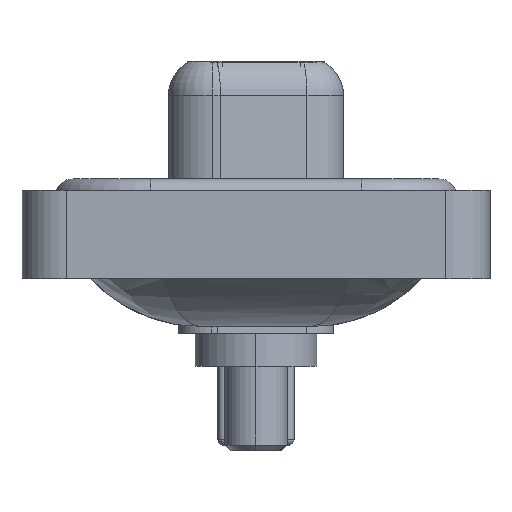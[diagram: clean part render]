
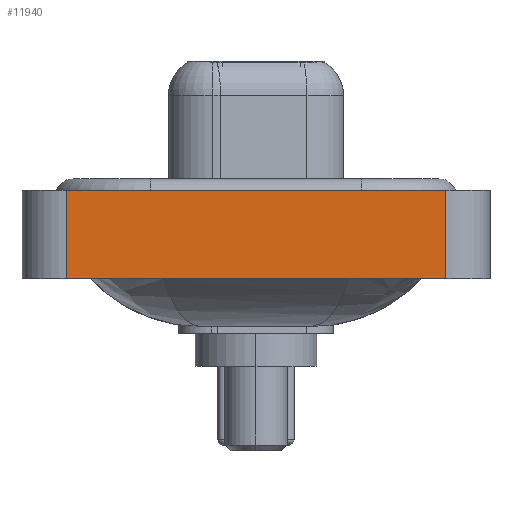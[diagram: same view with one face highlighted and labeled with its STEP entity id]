
A CAD part, left-side view. The second image highlights one B-rep face of the part: STEP entity #11940.
In plain terms, the highlighted planar face has unit normal (-1, 0, 0).
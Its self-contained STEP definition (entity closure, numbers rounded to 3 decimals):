
#289 = EDGE_CURVE ( 'NONE', #5348, #13883, #7500, .T. ) ;
#914 = CARTESIAN_POINT ( 'NONE',  ( -7.35, -8.55, 0.4 ) ) ;
#1150 = DIRECTION ( 'NONE',  ( -1., 0., 0. ) ) ;
#1490 = VECTOR ( 'NONE', #8801, 1000. ) ;
#3042 = DIRECTION ( 'NONE',  ( 0., 0., 1. ) ) ;
#4595 = ORIENTED_EDGE ( 'NONE', *, *, #289, .T. ) ;
#5348 = VERTEX_POINT ( 'NONE', #18067 ) ;
#5711 = VERTEX_POINT ( 'NONE', #15354 ) ;
#6177 = VECTOR ( 'NONE', #18657, 1000. ) ;
#6474 = EDGE_CURVE ( 'NONE', #13883, #6949, #16460, .T. ) ;
#6839 = ORIENTED_EDGE ( 'NONE', *, *, #17143, .F. ) ;
#6949 = VERTEX_POINT ( 'NONE', #914 ) ;
#7310 = DIRECTION ( 'NONE',  ( 0., 0., 1. ) ) ;
#7500 = LINE ( 'NONE', #20463, #8981 ) ;
#8801 = DIRECTION ( 'NONE',  ( 0., 0., 1. ) ) ;
#8981 = VECTOR ( 'NONE', #15478, 1000. ) ;
#9640 = VECTOR ( 'NONE', #7310, 1000. ) ;
#9641 = EDGE_CURVE ( 'NONE', #5711, #6949, #20261, .T. ) ;
#10365 = ORIENTED_EDGE ( 'NONE', *, *, #6474, .T. ) ;
#10560 = AXIS2_PLACEMENT_3D ( 'NONE', #10708, #1150, #3042 ) ;
#10708 = CARTESIAN_POINT ( 'NONE',  ( -7.35, -8.55, -3.6 ) ) ;
#10801 = PLANE ( 'NONE',  #10560 ) ;
#11940 = ADVANCED_FACE ( 'NONE', ( #19190 ), #10801, .T. ) ;
#12184 = CARTESIAN_POINT ( 'NONE',  ( -7.35, -8.55, 0.4 ) ) ;
#12291 = CARTESIAN_POINT ( 'NONE',  ( -7.35, 8.55, -3.6 ) ) ;
#12324 = EDGE_LOOP ( 'NONE', ( #10365, #17225, #6839, #4595 ) ) ;
#13771 = CARTESIAN_POINT ( 'NONE',  ( -7.35, -8.55, -3.6 ) ) ;
#13883 = VERTEX_POINT ( 'NONE', #13771 ) ;
#15354 = CARTESIAN_POINT ( 'NONE',  ( -7.35, 8.55, 0.4 ) ) ;
#15478 = DIRECTION ( 'NONE',  ( 0., -1., 0. ) ) ;
#16460 = LINE ( 'NONE', #19849, #1490 ) ;
#17072 = LINE ( 'NONE', #12291, #9640 ) ;
#17143 = EDGE_CURVE ( 'NONE', #5348, #5711, #17072, .T. ) ;
#17225 = ORIENTED_EDGE ( 'NONE', *, *, #9641, .F. ) ;
#18067 = CARTESIAN_POINT ( 'NONE',  ( -7.35, 8.55, -3.6 ) ) ;
#18657 = DIRECTION ( 'NONE',  ( 0., -1., 0. ) ) ;
#19190 = FACE_OUTER_BOUND ( 'NONE', #12324, .T. ) ;
#19849 = CARTESIAN_POINT ( 'NONE',  ( -7.35, -8.55, -3.6 ) ) ;
#20261 = LINE ( 'NONE', #12184, #6177 ) ;
#20463 = CARTESIAN_POINT ( 'NONE',  ( -7.35, -8.55, -3.6 ) ) ;
